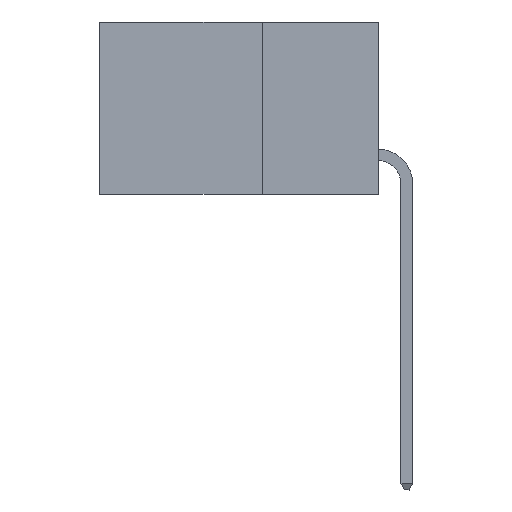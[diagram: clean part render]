
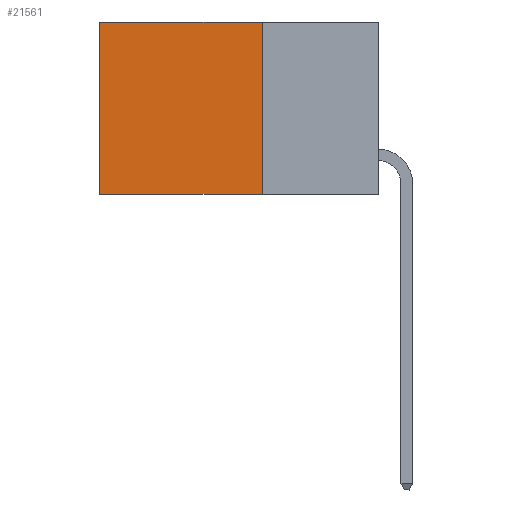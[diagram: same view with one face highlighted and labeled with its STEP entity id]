
A CAD part, left-side view. The second image highlights one B-rep face of the part: STEP entity #21561.
In plain terms, the highlighted planar face has unit normal (-1, 0, 0).
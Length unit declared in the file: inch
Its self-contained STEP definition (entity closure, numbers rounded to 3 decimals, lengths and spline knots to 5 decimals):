
#649 = CARTESIAN_POINT ( 'NONE',  ( 0.298, 0.25, 0. ) ) ;
#1661 = FACE_OUTER_BOUND ( 'NONE', #2321, .T. ) ;
#2321 = EDGE_LOOP ( 'NONE', ( #13535, #15826, #10403, #23529 ) ) ;
#2895 = VECTOR ( 'NONE', #26488, 39.37008 ) ;
#2982 = VECTOR ( 'NONE', #12631, 39.37008 ) ;
#3272 = VERTEX_POINT ( 'NONE', #17886 ) ;
#3510 = EDGE_CURVE ( 'NONE', #8339, #20262, #22061, .T. ) ;
#3819 = CARTESIAN_POINT ( 'NONE',  ( 0.298, 0.25, 0. ) ) ;
#4975 = CARTESIAN_POINT ( 'NONE',  ( 0.298, 0.25, 0. ) ) ;
#5106 = VECTOR ( 'NONE', #28776, 39.37008 ) ;
#5905 = AXIS2_PLACEMENT_3D ( 'NONE', #4975, #11349, #6801 ) ;
#6801 = DIRECTION ( 'NONE',  ( 0., 0., -1. ) ) ;
#8339 = VERTEX_POINT ( 'NONE', #9981 ) ;
#9981 = CARTESIAN_POINT ( 'NONE',  ( 0.298, 0.25, -0.37 ) ) ;
#10403 = ORIENTED_EDGE ( 'NONE', *, *, #28468, .F. ) ;
#11187 = CARTESIAN_POINT ( 'NONE',  ( 0.298, 0.6, -0.37 ) ) ;
#11209 = EDGE_CURVE ( 'NONE', #3272, #20262, #15713, .T. ) ;
#11349 = DIRECTION ( 'NONE',  ( 1., 0., 0. ) ) ;
#12631 = DIRECTION ( 'NONE',  ( 0., 0., -1. ) ) ;
#13201 = CARTESIAN_POINT ( 'NONE',  ( 0.298, 0.25, 0. ) ) ;
#13535 = ORIENTED_EDGE ( 'NONE', *, *, #11209, .T. ) ;
#13543 = DIRECTION ( 'NONE',  ( 0., 0., -1. ) ) ;
#13742 = CARTESIAN_POINT ( 'NONE',  ( 0.298, 0.6, 0. ) ) ;
#14309 = VECTOR ( 'NONE', #13543, 39.37008 ) ;
#15713 = LINE ( 'NONE', #13742, #14309 ) ;
#15826 = ORIENTED_EDGE ( 'NONE', *, *, #3510, .F. ) ;
#17886 = CARTESIAN_POINT ( 'NONE',  ( 0.298, 0.6, 0. ) ) ;
#20164 = PLANE ( 'NONE',  #5905 ) ;
#20262 = VERTEX_POINT ( 'NONE', #11187 ) ;
#21561 = ADVANCED_FACE ( 'NONE', ( #1661 ), #20164, .F. ) ;
#22061 = LINE ( 'NONE', #28571, #2895 ) ;
#23529 = ORIENTED_EDGE ( 'NONE', *, *, #26832, .T. ) ;
#23536 = LINE ( 'NONE', #3819, #2982 ) ;
#26488 = DIRECTION ( 'NONE',  ( 0., 1., 0. ) ) ;
#26832 = EDGE_CURVE ( 'NONE', #26925, #3272, #27049, .T. ) ;
#26925 = VERTEX_POINT ( 'NONE', #649 ) ;
#27049 = LINE ( 'NONE', #13201, #5106 ) ;
#28468 = EDGE_CURVE ( 'NONE', #26925, #8339, #23536, .T. ) ;
#28571 = CARTESIAN_POINT ( 'NONE',  ( 0.298, 0.25, -0.37 ) ) ;
#28776 = DIRECTION ( 'NONE',  ( 0., 1., 0. ) ) ;
